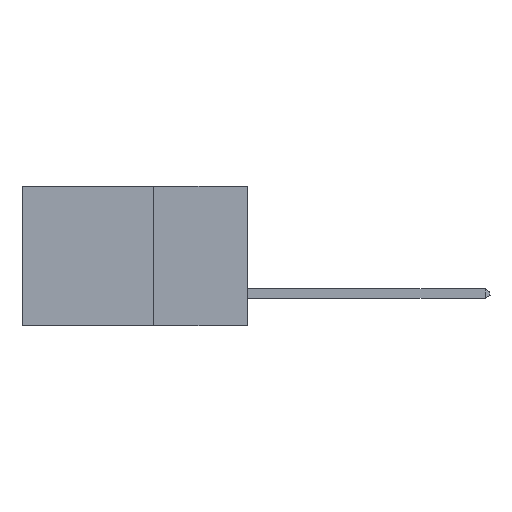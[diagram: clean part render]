
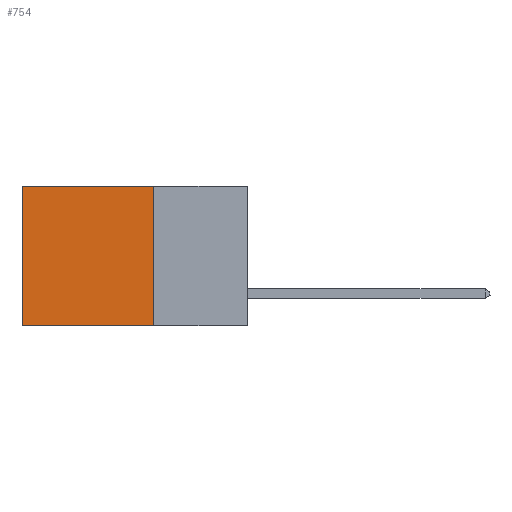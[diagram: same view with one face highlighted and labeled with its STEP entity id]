
A CAD part, left-side view. The second image highlights one B-rep face of the part: STEP entity #754.
In plain terms, the highlighted planar face has unit normal (-1, 0, 0).
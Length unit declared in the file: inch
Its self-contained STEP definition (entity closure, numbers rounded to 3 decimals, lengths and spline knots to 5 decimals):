
#63 = FACE_OUTER_BOUND ( 'NONE', #8138, .T. ) ;
#335 = LINE ( 'NONE', #5184, #5479 ) ;
#754 = ADVANCED_FACE ( 'NONE', ( #63 ), #9782, .F. ) ;
#1044 = DIRECTION ( 'NONE',  ( 0., 1., 0. ) ) ;
#1737 = VERTEX_POINT ( 'NONE', #6869 ) ;
#2548 = VERTEX_POINT ( 'NONE', #14197 ) ;
#3323 = LINE ( 'NONE', #11096, #12289 ) ;
#3427 = DIRECTION ( 'NONE',  ( 0., 1., 0. ) ) ;
#3815 = DIRECTION ( 'NONE',  ( 1., 0., 0. ) ) ;
#4323 = CARTESIAN_POINT ( 'NONE',  ( 0.298, 0.6, 0. ) ) ;
#4449 = CARTESIAN_POINT ( 'NONE',  ( 0.298, 0.6, -0.37 ) ) ;
#5184 = CARTESIAN_POINT ( 'NONE',  ( 0.298, 0.25, 0. ) ) ;
#5479 = VECTOR ( 'NONE', #12310, 39.37008 ) ;
#5926 = EDGE_CURVE ( 'NONE', #9543, #15025, #3323, .T. ) ;
#5988 = VECTOR ( 'NONE', #3427, 39.37008 ) ;
#6115 = VECTOR ( 'NONE', #1044, 39.37008 ) ;
#6211 = CARTESIAN_POINT ( 'NONE',  ( 0.298, 0.25, 0. ) ) ;
#6701 = AXIS2_PLACEMENT_3D ( 'NONE', #6211, #3815, #11005 ) ;
#6869 = CARTESIAN_POINT ( 'NONE',  ( 0.298, 0.25, 0. ) ) ;
#7380 = ORIENTED_EDGE ( 'NONE', *, *, #7906, .F. ) ;
#7906 = EDGE_CURVE ( 'NONE', #2548, #15025, #14058, .T. ) ;
#8138 = EDGE_LOOP ( 'NONE', ( #10742, #7380, #11929, #14748 ) ) ;
#8778 = LINE ( 'NONE', #10331, #5988 ) ;
#9543 = VERTEX_POINT ( 'NONE', #4323 ) ;
#9782 = PLANE ( 'NONE',  #6701 ) ;
#10331 = CARTESIAN_POINT ( 'NONE',  ( 0.298, 0.25, 0. ) ) ;
#10742 = ORIENTED_EDGE ( 'NONE', *, *, #5926, .T. ) ;
#11005 = DIRECTION ( 'NONE',  ( 0., 0., -1. ) ) ;
#11096 = CARTESIAN_POINT ( 'NONE',  ( 0.298, 0.6, 0. ) ) ;
#11279 = CARTESIAN_POINT ( 'NONE',  ( 0.298, 0.25, -0.37 ) ) ;
#11300 = DIRECTION ( 'NONE',  ( 0., 0., -1. ) ) ;
#11320 = EDGE_CURVE ( 'NONE', #1737, #2548, #335, .T. ) ;
#11929 = ORIENTED_EDGE ( 'NONE', *, *, #11320, .F. ) ;
#12289 = VECTOR ( 'NONE', #11300, 39.37008 ) ;
#12310 = DIRECTION ( 'NONE',  ( 0., 0., -1. ) ) ;
#14058 = LINE ( 'NONE', #11279, #6115 ) ;
#14197 = CARTESIAN_POINT ( 'NONE',  ( 0.298, 0.25, -0.37 ) ) ;
#14742 = EDGE_CURVE ( 'NONE', #1737, #9543, #8778, .T. ) ;
#14748 = ORIENTED_EDGE ( 'NONE', *, *, #14742, .T. ) ;
#15025 = VERTEX_POINT ( 'NONE', #4449 ) ;
